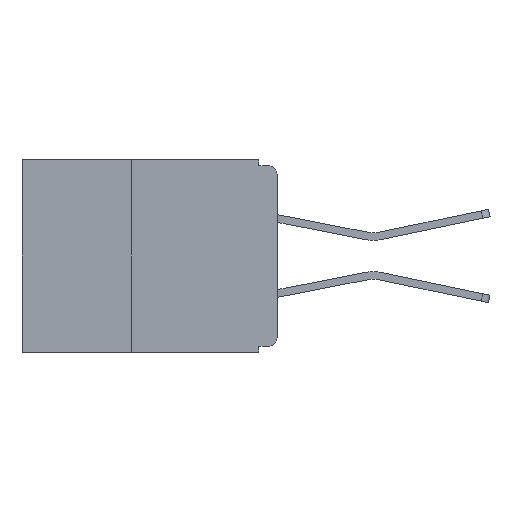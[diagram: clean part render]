
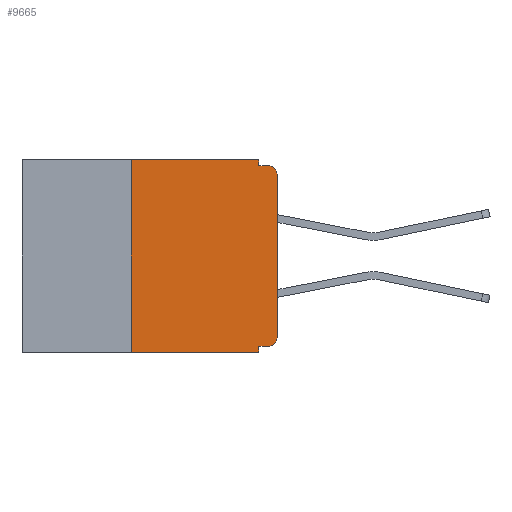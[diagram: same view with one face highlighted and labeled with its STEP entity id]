
A CAD part, left-side view. The second image highlights one B-rep face of the part: STEP entity #9665.
In plain terms, the highlighted planar face has unit normal (-1, 0, 0).
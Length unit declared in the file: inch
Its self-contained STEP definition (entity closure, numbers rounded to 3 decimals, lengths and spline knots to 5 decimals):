
#583 = LINE ( 'NONE', #20398, #14669 ) ;
#1908 = EDGE_CURVE ( 'NONE', #5129, #12785, #32913, .T. ) ;
#1975 = DIRECTION ( 'NONE',  ( 0., -1., 0. ) ) ;
#2153 = VERTEX_POINT ( 'NONE', #22336 ) ;
#3038 = EDGE_CURVE ( 'NONE', #20392, #13728, #24408, .T. ) ;
#3454 = CARTESIAN_POINT ( 'NONE',  ( 0., 0.031, -0.33 ) ) ;
#3547 = CARTESIAN_POINT ( 'NONE',  ( 0., 0.031, -0.01 ) ) ;
#3882 = DIRECTION ( 'NONE',  ( 0., 0., 1. ) ) ;
#4136 = ORIENTED_EDGE ( 'NONE', *, *, #26793, .F. ) ;
#4478 = CARTESIAN_POINT ( 'NONE',  ( 0., 0.25, -0.33 ) ) ;
#4494 = EDGE_LOOP ( 'NONE', ( #12372, #27814, #14816, #22983, #18517, #13234, #8659, #4136, #12366, #30244 ) ) ;
#4606 = LINE ( 'NONE', #27186, #31543 ) ;
#4785 = CARTESIAN_POINT ( 'NONE',  ( 0., 0.031, -0.32 ) ) ;
#4864 = CARTESIAN_POINT ( 'NONE',  ( 0., 0., -0.025 ) ) ;
#4942 = CARTESIAN_POINT ( 'NONE',  ( 0., 0.437, 0. ) ) ;
#5129 = VERTEX_POINT ( 'NONE', #31461 ) ;
#5149 = CARTESIAN_POINT ( 'NONE',  ( 0., 0.031, 0. ) ) ;
#5260 = VECTOR ( 'NONE', #8468, 39.37008 ) ;
#5294 = DIRECTION ( 'NONE',  ( -1., 0., 0. ) ) ;
#5609 = DIRECTION ( 'NONE',  ( -1., 0., 0. ) ) ;
#5654 = VERTEX_POINT ( 'NONE', #28711 ) ;
#6329 = VECTOR ( 'NONE', #32407, 39.37008 ) ;
#6379 = EDGE_CURVE ( 'NONE', #12785, #2153, #32975, .T. ) ;
#7568 = DIRECTION ( 'NONE',  ( 0., 0., -1. ) ) ;
#8319 = CIRCLE ( 'NONE', #31746, 0.015 ) ;
#8468 = DIRECTION ( 'NONE',  ( 0., -1., 0. ) ) ;
#8659 = ORIENTED_EDGE ( 'NONE', *, *, #20322, .T. ) ;
#8905 = VECTOR ( 'NONE', #10486, 39.37008 ) ;
#8995 = CARTESIAN_POINT ( 'NONE',  ( 0., 0., 0. ) ) ;
#9665 = ADVANCED_FACE ( 'NONE', ( #15370 ), #18047, .F. ) ;
#10230 = CARTESIAN_POINT ( 'NONE',  ( 0., 0.015, -0.32 ) ) ;
#10486 = DIRECTION ( 'NONE',  ( 0., 0., -1. ) ) ;
#10700 = CARTESIAN_POINT ( 'NONE',  ( 0., 0.031, -0.33 ) ) ;
#11698 = AXIS2_PLACEMENT_3D ( 'NONE', #21007, #5294, #23599 ) ;
#12366 = ORIENTED_EDGE ( 'NONE', *, *, #3038, .F. ) ;
#12372 = ORIENTED_EDGE ( 'NONE', *, *, #21392, .T. ) ;
#12785 = VERTEX_POINT ( 'NONE', #3547 ) ;
#13086 = DIRECTION ( 'NONE',  ( 0., 1., 0. ) ) ;
#13202 = VERTEX_POINT ( 'NONE', #10700 ) ;
#13234 = ORIENTED_EDGE ( 'NONE', *, *, #23736, .F. ) ;
#13375 = LINE ( 'NONE', #8995, #6329 ) ;
#13728 = VERTEX_POINT ( 'NONE', #4785 ) ;
#14234 = DIRECTION ( 'NONE',  ( 0., -1., 0. ) ) ;
#14669 = VECTOR ( 'NONE', #1975, 39.37008 ) ;
#14816 = ORIENTED_EDGE ( 'NONE', *, *, #6379, .F. ) ;
#15126 = EDGE_CURVE ( 'NONE', #21005, #2153, #8319, .T. ) ;
#15370 = FACE_OUTER_BOUND ( 'NONE', #4494, .T. ) ;
#15740 = VECTOR ( 'NONE', #3882, 39.37008 ) ;
#16584 = LINE ( 'NONE', #24842, #15740 ) ;
#17569 = AXIS2_PLACEMENT_3D ( 'NONE', #4942, #23251, #7568 ) ;
#18047 = PLANE ( 'NONE',  #17569 ) ;
#18517 = ORIENTED_EDGE ( 'NONE', *, *, #24337, .F. ) ;
#20322 = EDGE_CURVE ( 'NONE', #33353, #13202, #583, .T. ) ;
#20392 = VERTEX_POINT ( 'NONE', #10230 ) ;
#20398 = CARTESIAN_POINT ( 'NONE',  ( 0., 0.437, -0.33 ) ) ;
#21005 = VERTEX_POINT ( 'NONE', #4864 ) ;
#21007 = CARTESIAN_POINT ( 'NONE',  ( 0., 0.015, -0.305 ) ) ;
#21332 = CARTESIAN_POINT ( 'NONE',  ( 0., 0.015, -0.025 ) ) ;
#21392 = EDGE_CURVE ( 'NONE', #5654, #21005, #13375, .T. ) ;
#21565 = EDGE_CURVE ( 'NONE', #20392, #5654, #23929, .T. ) ;
#22336 = CARTESIAN_POINT ( 'NONE',  ( 0., 0.015, -0.01 ) ) ;
#22983 = ORIENTED_EDGE ( 'NONE', *, *, #1908, .F. ) ;
#23251 = DIRECTION ( 'NONE',  ( 1., 0., 0. ) ) ;
#23336 = VERTEX_POINT ( 'NONE', #28377 ) ;
#23588 = VECTOR ( 'NONE', #13086, 39.37008 ) ;
#23599 = DIRECTION ( 'NONE',  ( 0., 0., -1. ) ) ;
#23736 = EDGE_CURVE ( 'NONE', #33353, #23336, #16584, .T. ) ;
#23924 = DIRECTION ( 'NONE',  ( 0., 0., -1. ) ) ;
#23929 = CIRCLE ( 'NONE', #11698, 0.015 ) ;
#24337 = EDGE_CURVE ( 'NONE', #23336, #5129, #4606, .T. ) ;
#24408 = LINE ( 'NONE', #31214, #23588 ) ;
#24532 = VECTOR ( 'NONE', #27051, 39.37008 ) ;
#24842 = CARTESIAN_POINT ( 'NONE',  ( 0., 0.25, -0.33 ) ) ;
#26764 = CARTESIAN_POINT ( 'NONE',  ( 0., 0., -0.01 ) ) ;
#26793 = EDGE_CURVE ( 'NONE', #13728, #13202, #31420, .T. ) ;
#27051 = DIRECTION ( 'NONE',  ( 0., 0., -1. ) ) ;
#27186 = CARTESIAN_POINT ( 'NONE',  ( 0., 0.437, 0. ) ) ;
#27814 = ORIENTED_EDGE ( 'NONE', *, *, #15126, .T. ) ;
#28377 = CARTESIAN_POINT ( 'NONE',  ( 0., 0.25, 0. ) ) ;
#28711 = CARTESIAN_POINT ( 'NONE',  ( 0., 0., -0.305 ) ) ;
#30244 = ORIENTED_EDGE ( 'NONE', *, *, #21565, .T. ) ;
#31214 = CARTESIAN_POINT ( 'NONE',  ( 0., 0., -0.32 ) ) ;
#31420 = LINE ( 'NONE', #3454, #24532 ) ;
#31461 = CARTESIAN_POINT ( 'NONE',  ( 0., 0.031, 0. ) ) ;
#31543 = VECTOR ( 'NONE', #14234, 39.37008 ) ;
#31746 = AXIS2_PLACEMENT_3D ( 'NONE', #21332, #5609, #23924 ) ;
#32407 = DIRECTION ( 'NONE',  ( 0., 0., 1. ) ) ;
#32913 = LINE ( 'NONE', #5149, #8905 ) ;
#32975 = LINE ( 'NONE', #26764, #5260 ) ;
#33353 = VERTEX_POINT ( 'NONE', #4478 ) ;
